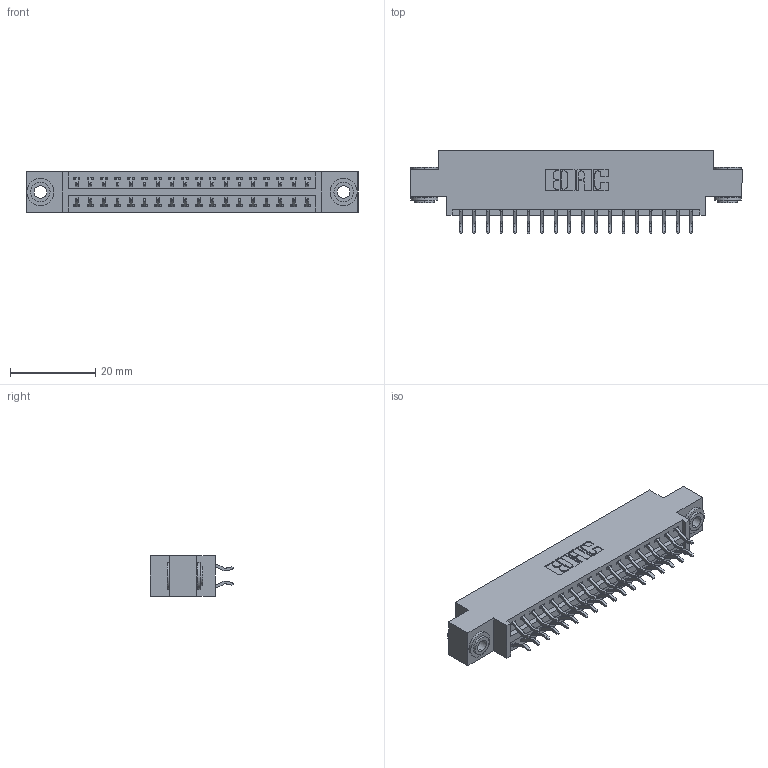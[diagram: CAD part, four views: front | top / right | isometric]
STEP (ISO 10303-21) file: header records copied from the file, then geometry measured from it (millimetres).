
FILE_DESCRIPTION (( 'STEP AP203' ), '1' );
FILE_NAME ('346-036-556-803.STEP', '2018-08-24T02:23:01', ( '' ), ( '' ), 'SwSTEP 2.0', 'SolidWorks 2016', '' );
FILE_SCHEMA (( 'CONFIG_CONTROL_DESIGN' ));
Length unit declared in the file: inch
Products named in the file (4): 346 Part_0.170 Offset - 0.156 Dia-TH; 345-292-001_556 Tail; 345-250-002_345-250-002-102; 346-036-556-803
Assembly tree (39 placements, depth 2):
  346-036-556-803
    346 Part_0.170 Offset - 0.156 Dia-TH
    345-292-001_556 Tail  x36
    345-250-002_345-250-002-102  x2
Bounding box: 77.72 x 19.57 x 9.4 mm (x, y, z)
Volume: 7256 mm3; surface area: 9957 mm2
Topology: 39 solids, 39 shells, 2252 faces, 6645 edges, 4378 vertices
Faces by surface type: plane 1494, cylinder 750, cone 8
Entity records: 15980 total; most frequent: CARTESIAN_POINT 2659, ORIENTED_EDGE 2574, DIRECTION 2413, EDGE_CURVE 1287, LINE 1051, VECTOR 1051, VERTEX_POINT 854, AXIS2_PLACEMENT_3D 681
